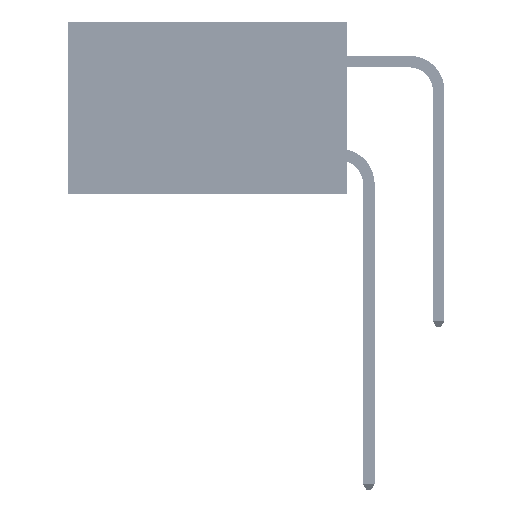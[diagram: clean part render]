
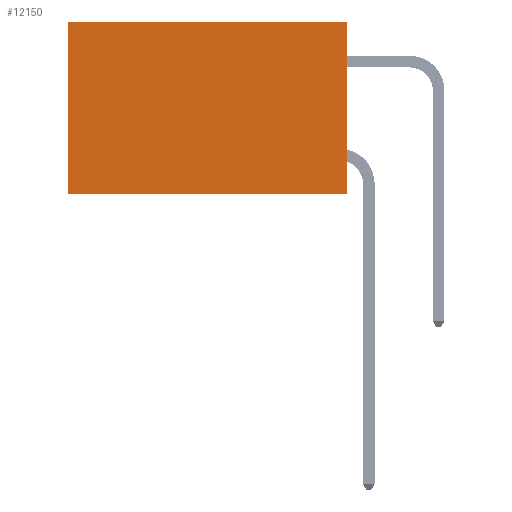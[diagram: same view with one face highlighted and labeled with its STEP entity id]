
A CAD part, left-side view. The second image highlights one B-rep face of the part: STEP entity #12150.
In plain terms, the highlighted planar face has unit normal (-1, 0, 0).
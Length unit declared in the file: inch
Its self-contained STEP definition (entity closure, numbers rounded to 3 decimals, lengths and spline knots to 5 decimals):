
#394 = FACE_OUTER_BOUND ( 'NONE', #26422, .T. ) ;
#1850 = VECTOR ( 'NONE', #43787, 39.37008 ) ;
#2358 = EDGE_CURVE ( 'NONE', #38827, #6791, #33991, .T. ) ;
#3553 = LINE ( 'NONE', #13472, #30429 ) ;
#3684 = DIRECTION ( 'NONE',  ( 0., 0., -1. ) ) ;
#3974 = CARTESIAN_POINT ( 'NONE',  ( 0.2875, 0.6, -0.37 ) ) ;
#4035 = DIRECTION ( 'NONE',  ( 1., 0., 0. ) ) ;
#5485 = DIRECTION ( 'NONE',  ( 0., 1., 0. ) ) ;
#5552 = VECTOR ( 'NONE', #36832, 39.37008 ) ;
#6791 = VERTEX_POINT ( 'NONE', #12008 ) ;
#7498 = DIRECTION ( 'NONE',  ( 0., 0., -1. ) ) ;
#9473 = CARTESIAN_POINT ( 'NONE',  ( 0.2875, 0.6, 0. ) ) ;
#10316 = CARTESIAN_POINT ( 'NONE',  ( 0.2875, 0., 0. ) ) ;
#10751 = EDGE_CURVE ( 'NONE', #6791, #43962, #3553, .T. ) ;
#12008 = CARTESIAN_POINT ( 'NONE',  ( 0.2875, 0., -0.37 ) ) ;
#12150 = ADVANCED_FACE ( 'NONE', ( #394 ), #38875, .F. ) ;
#13472 = CARTESIAN_POINT ( 'NONE',  ( 0.2875, 0., -0.37 ) ) ;
#15004 = VECTOR ( 'NONE', #7498, 39.37008 ) ;
#15449 = VERTEX_POINT ( 'NONE', #22957 ) ;
#16259 = CARTESIAN_POINT ( 'NONE',  ( 0.2875, 0., 0. ) ) ;
#22558 = LINE ( 'NONE', #39845, #1850 ) ;
#22957 = CARTESIAN_POINT ( 'NONE',  ( 0.2875, 0.6, 0. ) ) ;
#25361 = EDGE_CURVE ( 'NONE', #15449, #43962, #47138, .T. ) ;
#26422 = EDGE_LOOP ( 'NONE', ( #47890, #28200, #33248, #41076 ) ) ;
#28200 = ORIENTED_EDGE ( 'NONE', *, *, #10751, .F. ) ;
#30429 = VECTOR ( 'NONE', #5485, 39.37008 ) ;
#33248 = ORIENTED_EDGE ( 'NONE', *, *, #2358, .F. ) ;
#33991 = LINE ( 'NONE', #10316, #15004 ) ;
#36832 = DIRECTION ( 'NONE',  ( 0., 0., -1. ) ) ;
#38827 = VERTEX_POINT ( 'NONE', #16259 ) ;
#38875 = PLANE ( 'NONE',  #46408 ) ;
#39845 = CARTESIAN_POINT ( 'NONE',  ( 0.2875, 0., 0. ) ) ;
#41076 = ORIENTED_EDGE ( 'NONE', *, *, #47072, .T. ) ;
#43787 = DIRECTION ( 'NONE',  ( 0., 1., 0. ) ) ;
#43962 = VERTEX_POINT ( 'NONE', #3974 ) ;
#46408 = AXIS2_PLACEMENT_3D ( 'NONE', #46734, #4035, #3684 ) ;
#46734 = CARTESIAN_POINT ( 'NONE',  ( 0.2875, 0., 0. ) ) ;
#47072 = EDGE_CURVE ( 'NONE', #38827, #15449, #22558, .T. ) ;
#47138 = LINE ( 'NONE', #9473, #5552 ) ;
#47890 = ORIENTED_EDGE ( 'NONE', *, *, #25361, .T. ) ;
